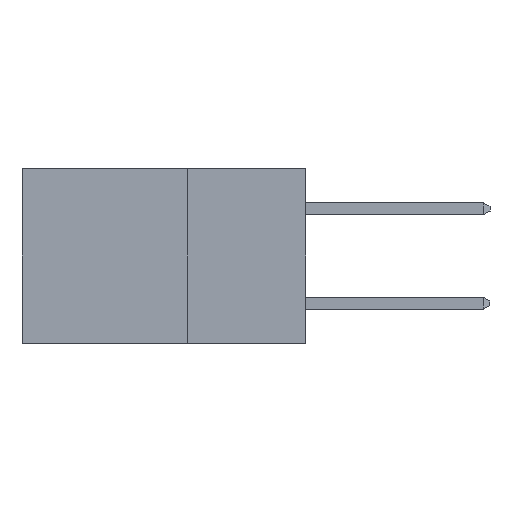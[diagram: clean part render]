
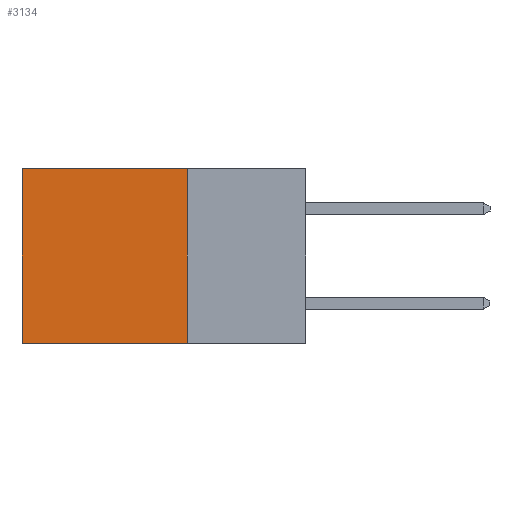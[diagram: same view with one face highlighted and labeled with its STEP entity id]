
A CAD part, left-side view. The second image highlights one B-rep face of the part: STEP entity #3134.
In plain terms, the highlighted planar face has unit normal (-1, 0, 0).
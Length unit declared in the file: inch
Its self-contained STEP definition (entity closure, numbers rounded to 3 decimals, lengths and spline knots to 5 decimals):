
#653 = VECTOR ( 'NONE', #5683, 39.37008 ) ;
#1077 = CARTESIAN_POINT ( 'NONE',  ( 0.298, 0.25, 0. ) ) ;
#2277 = CARTESIAN_POINT ( 'NONE',  ( 0.298, 0.6, -0.37 ) ) ;
#3007 = CARTESIAN_POINT ( 'NONE',  ( 0.298, 0.25, 0. ) ) ;
#3134 = ADVANCED_FACE ( 'NONE', ( #11374 ), #4109, .F. ) ;
#4042 = VERTEX_POINT ( 'NONE', #2277 ) ;
#4109 = PLANE ( 'NONE',  #4289 ) ;
#4116 = DIRECTION ( 'NONE',  ( 1., 0., 0. ) ) ;
#4289 = AXIS2_PLACEMENT_3D ( 'NONE', #5260, #4116, #12456 ) ;
#4430 = VECTOR ( 'NONE', #9647, 39.37008 ) ;
#5260 = CARTESIAN_POINT ( 'NONE',  ( 0.298, 0.25, 0. ) ) ;
#5640 = CARTESIAN_POINT ( 'NONE',  ( 0.298, 0.25, -0.37 ) ) ;
#5683 = DIRECTION ( 'NONE',  ( 0., 0., -1. ) ) ;
#5783 = ORIENTED_EDGE ( 'NONE', *, *, #12377, .T. ) ;
#6195 = ORIENTED_EDGE ( 'NONE', *, *, #8024, .F. ) ;
#6415 = LINE ( 'NONE', #9536, #13726 ) ;
#6538 = ORIENTED_EDGE ( 'NONE', *, *, #10853, .F. ) ;
#6832 = ORIENTED_EDGE ( 'NONE', *, *, #6917, .T. ) ;
#6917 = EDGE_CURVE ( 'NONE', #11289, #12769, #10153, .T. ) ;
#7431 = DIRECTION ( 'NONE',  ( 0., 0., -1. ) ) ;
#8024 = EDGE_CURVE ( 'NONE', #10828, #4042, #8032, .T. ) ;
#8032 = LINE ( 'NONE', #12695, #10769 ) ;
#8105 = EDGE_LOOP ( 'NONE', ( #5783, #6195, #6538, #6832 ) ) ;
#8618 = DIRECTION ( 'NONE',  ( 0., 1., 0. ) ) ;
#9536 = CARTESIAN_POINT ( 'NONE',  ( 0.298, 0.6, 0. ) ) ;
#9647 = DIRECTION ( 'NONE',  ( 0., 1., 0. ) ) ;
#10153 = LINE ( 'NONE', #1077, #4430 ) ;
#10190 = CARTESIAN_POINT ( 'NONE',  ( 0.298, 0.6, 0. ) ) ;
#10769 = VECTOR ( 'NONE', #8618, 39.37008 ) ;
#10828 = VERTEX_POINT ( 'NONE', #5640 ) ;
#10853 = EDGE_CURVE ( 'NONE', #11289, #10828, #12157, .T. ) ;
#10954 = CARTESIAN_POINT ( 'NONE',  ( 0.298, 0.25, 0. ) ) ;
#11289 = VERTEX_POINT ( 'NONE', #3007 ) ;
#11374 = FACE_OUTER_BOUND ( 'NONE', #8105, .T. ) ;
#12157 = LINE ( 'NONE', #10954, #653 ) ;
#12377 = EDGE_CURVE ( 'NONE', #12769, #4042, #6415, .T. ) ;
#12456 = DIRECTION ( 'NONE',  ( 0., 0., -1. ) ) ;
#12695 = CARTESIAN_POINT ( 'NONE',  ( 0.298, 0.25, -0.37 ) ) ;
#12769 = VERTEX_POINT ( 'NONE', #10190 ) ;
#13726 = VECTOR ( 'NONE', #7431, 39.37008 ) ;
